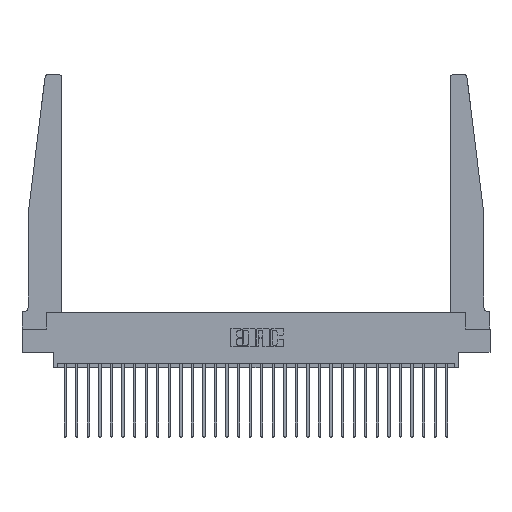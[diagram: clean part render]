
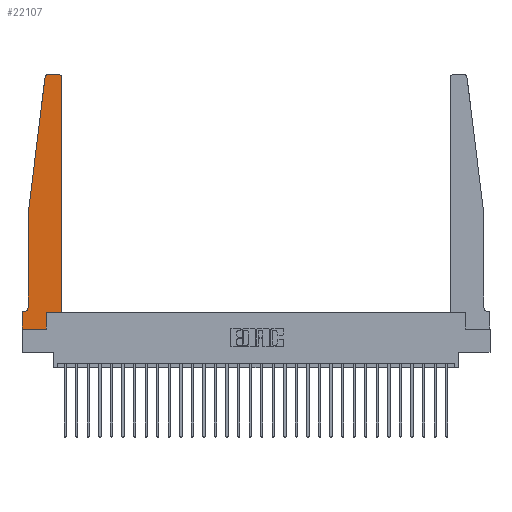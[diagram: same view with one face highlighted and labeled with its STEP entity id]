
A CAD part, top view. The second image highlights one B-rep face of the part: STEP entity #22107.
In plain terms, the highlighted planar face has unit normal (0, 0, 1).
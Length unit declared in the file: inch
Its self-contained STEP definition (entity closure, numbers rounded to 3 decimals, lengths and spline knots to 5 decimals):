
#262 = VERTEX_POINT ( 'NONE', #21662 ) ;
#724 = DIRECTION ( 'NONE',  ( 0., 0., -1. ) ) ;
#1283 = VECTOR ( 'NONE', #9118, 39.37008 ) ;
#1319 = CARTESIAN_POINT ( 'NONE',  ( 0.425, 0.18, 0.37 ) ) ;
#1551 = VECTOR ( 'NONE', #20176, 39.37008 ) ;
#1653 = CIRCLE ( 'NONE', #17897, 0.03 ) ;
#2287 = CARTESIAN_POINT ( 'NONE',  ( 0.425, 0.18, 0.37 ) ) ;
#2623 = EDGE_CURVE ( 'NONE', #11223, #9878, #7058, .T. ) ;
#3074 = ORIENTED_EDGE ( 'NONE', *, *, #16276, .T. ) ;
#3439 = LINE ( 'NONE', #27932, #18527 ) ;
#3899 = VERTEX_POINT ( 'NONE', #20298 ) ;
#3923 = CARTESIAN_POINT ( 'NONE',  ( 0.065, 1.25, 0.37 ) ) ;
#4147 = FACE_OUTER_BOUND ( 'NONE', #27017, .T. ) ;
#4292 = DIRECTION ( 'NONE',  ( -1., 0., 0. ) ) ;
#4382 = VECTOR ( 'NONE', #28266, 39.37008 ) ;
#4562 = VECTOR ( 'NONE', #27119, 39.37008 ) ;
#4894 = EDGE_CURVE ( 'NONE', #3899, #12848, #21574, .T. ) ;
#5672 = ORIENTED_EDGE ( 'NONE', *, *, #16887, .T. ) ;
#5782 = ORIENTED_EDGE ( 'NONE', *, *, #15178, .T. ) ;
#6183 = EDGE_CURVE ( 'NONE', #27841, #262, #23790, .T. ) ;
#6618 = CARTESIAN_POINT ( 'NONE',  ( 0., 0.1875, 0.37 ) ) ;
#7058 = CIRCLE ( 'NONE', #11235, 0.03 ) ;
#7682 = DIRECTION ( 'NONE',  ( -1., 0., 0. ) ) ;
#8371 = VERTEX_POINT ( 'NONE', #23908 ) ;
#8520 = PLANE ( 'NONE',  #11350 ) ;
#8958 = DIRECTION ( 'NONE',  ( 0., -1., 0. ) ) ;
#9078 = CARTESIAN_POINT ( 'NONE',  ( 0.27653, 2.75, 0.37 ) ) ;
#9118 = DIRECTION ( 'NONE',  ( 0., 1., 0. ) ) ;
#9304 = EDGE_CURVE ( 'NONE', #8371, #27841, #22900, .T. ) ;
#9561 = ORIENTED_EDGE ( 'NONE', *, *, #9304, .T. ) ;
#9772 = CARTESIAN_POINT ( 'NONE',  ( 0.015, 0.1875, 0.37 ) ) ;
#9878 = VERTEX_POINT ( 'NONE', #20741 ) ;
#10248 = ORIENTED_EDGE ( 'NONE', *, *, #12047, .T. ) ;
#10390 = ORIENTED_EDGE ( 'NONE', *, *, #2623, .T. ) ;
#10441 = CARTESIAN_POINT ( 'NONE',  ( 0.065, 0.1875, 0.37 ) ) ;
#10687 = ORIENTED_EDGE ( 'NONE', *, *, #6183, .T. ) ;
#10747 = VERTEX_POINT ( 'NONE', #9772 ) ;
#11015 = LINE ( 'NONE', #20310, #1283 ) ;
#11223 = VERTEX_POINT ( 'NONE', #21425 ) ;
#11235 = AXIS2_PLACEMENT_3D ( 'NONE', #19677, #15317, #24129 ) ;
#11350 = AXIS2_PLACEMENT_3D ( 'NONE', #6618, #28498, #13300 ) ;
#11377 = DIRECTION ( 'NONE',  ( 1., 0., 0. ) ) ;
#12047 = EDGE_CURVE ( 'NONE', #10747, #3899, #12605, .T. ) ;
#12605 = LINE ( 'NONE', #10441, #19700 ) ;
#12848 = VERTEX_POINT ( 'NONE', #27855 ) ;
#13276 = VECTOR ( 'NONE', #14287, 39.37008 ) ;
#13300 = DIRECTION ( 'NONE',  ( 1., 0., 0. ) ) ;
#13582 = CARTESIAN_POINT ( 'NONE',  ( 0.2605, 0.18, 0.37 ) ) ;
#14234 = VERTEX_POINT ( 'NONE', #28041 ) ;
#14240 = CARTESIAN_POINT ( 'NONE',  ( 0.015, 0.2375, 0.37 ) ) ;
#14287 = DIRECTION ( 'NONE',  ( 1., 0., 0. ) ) ;
#14784 = EDGE_CURVE ( 'NONE', #24383, #11223, #15962, .T. ) ;
#14974 = CARTESIAN_POINT ( 'NONE',  ( 0.425, 0.18, 0.37 ) ) ;
#15178 = EDGE_CURVE ( 'NONE', #9878, #27952, #19710, .T. ) ;
#15317 = DIRECTION ( 'NONE',  ( 0., 0., 1. ) ) ;
#15343 = CARTESIAN_POINT ( 'NONE',  ( 0.25, 2.75, 0.37 ) ) ;
#15627 = ORIENTED_EDGE ( 'NONE', *, *, #14784, .T. ) ;
#15761 = ORIENTED_EDGE ( 'NONE', *, *, #4894, .T. ) ;
#15962 = LINE ( 'NONE', #2287, #1551 ) ;
#15974 = ORIENTED_EDGE ( 'NONE', *, *, #23287, .T. ) ;
#16276 = EDGE_CURVE ( 'NONE', #27952, #8371, #1653, .T. ) ;
#16887 = EDGE_CURVE ( 'NONE', #262, #10747, #23474, .T. ) ;
#17201 = EDGE_CURVE ( 'NONE', #14234, #18966, #11015, .T. ) ;
#17897 = AXIS2_PLACEMENT_3D ( 'NONE', #26702, #22779, #11377 ) ;
#17973 = ORIENTED_EDGE ( 'NONE', *, *, #22774, .T. ) ;
#18527 = VECTOR ( 'NONE', #25624, 39.37008 ) ;
#18966 = VERTEX_POINT ( 'NONE', #13582 ) ;
#19677 = CARTESIAN_POINT ( 'NONE',  ( 0.395, 2.72, 0.37 ) ) ;
#19700 = VECTOR ( 'NONE', #21444, 39.37008 ) ;
#19710 = LINE ( 'NONE', #15343, #21905 ) ;
#20176 = DIRECTION ( 'NONE',  ( 0., 1., 0. ) ) ;
#20298 = CARTESIAN_POINT ( 'NONE',  ( 0., 0.1875, 0.37 ) ) ;
#20310 = CARTESIAN_POINT ( 'NONE',  ( 0.2605, 0.18, 0.37 ) ) ;
#20741 = CARTESIAN_POINT ( 'NONE',  ( 0.395, 2.75, 0.37 ) ) ;
#20755 = AXIS2_PLACEMENT_3D ( 'NONE', #14240, #724, #7682 ) ;
#21425 = CARTESIAN_POINT ( 'NONE',  ( 0.425, 2.72, 0.37 ) ) ;
#21444 = DIRECTION ( 'NONE',  ( -1., 0., 0. ) ) ;
#21574 = LINE ( 'NONE', #21713, #24575 ) ;
#21662 = CARTESIAN_POINT ( 'NONE',  ( 0.065, 0.2375, 0.37 ) ) ;
#21713 = CARTESIAN_POINT ( 'NONE',  ( 0., 0., 0.37 ) ) ;
#21882 = ORIENTED_EDGE ( 'NONE', *, *, #17201, .T. ) ;
#21905 = VECTOR ( 'NONE', #4292, 39.37008 ) ;
#22107 = ADVANCED_FACE ( 'NONE', ( #4147 ), #8520, .T. ) ;
#22774 = EDGE_CURVE ( 'NONE', #18966, #24383, #27586, .T. ) ;
#22779 = DIRECTION ( 'NONE',  ( 0., 0., 1. ) ) ;
#22900 = LINE ( 'NONE', #25102, #4562 ) ;
#23287 = EDGE_CURVE ( 'NONE', #12848, #14234, #3439, .T. ) ;
#23474 = CIRCLE ( 'NONE', #20755, 0.05 ) ;
#23790 = LINE ( 'NONE', #3923, #4382 ) ;
#23908 = CARTESIAN_POINT ( 'NONE',  ( 0.24675, 2.72367, 0.37 ) ) ;
#24129 = DIRECTION ( 'NONE',  ( 1., 0., 0. ) ) ;
#24383 = VERTEX_POINT ( 'NONE', #1319 ) ;
#24437 = CARTESIAN_POINT ( 'NONE',  ( 0.065, 1.25, 0.37 ) ) ;
#24575 = VECTOR ( 'NONE', #8958, 39.37008 ) ;
#25102 = CARTESIAN_POINT ( 'NONE',  ( 0.065, 1.25, 0.37 ) ) ;
#25624 = DIRECTION ( 'NONE',  ( 1., 0., 0. ) ) ;
#26702 = CARTESIAN_POINT ( 'NONE',  ( 0.27653, 2.72, 0.37 ) ) ;
#27017 = EDGE_LOOP ( 'NONE', ( #5782, #3074, #9561, #10687, #5672, #10248, #15761, #15974, #21882, #17973, #15627, #10390 ) ) ;
#27119 = DIRECTION ( 'NONE',  ( -0.122, -0.992, 0. ) ) ;
#27586 = LINE ( 'NONE', #14974, #13276 ) ;
#27841 = VERTEX_POINT ( 'NONE', #24437 ) ;
#27855 = CARTESIAN_POINT ( 'NONE',  ( 0., 0., 0.37 ) ) ;
#27932 = CARTESIAN_POINT ( 'NONE',  ( 0., 0., 0.37 ) ) ;
#27952 = VERTEX_POINT ( 'NONE', #9078 ) ;
#28041 = CARTESIAN_POINT ( 'NONE',  ( 0.2605, 0., 0.37 ) ) ;
#28266 = DIRECTION ( 'NONE',  ( 0., -1., 0. ) ) ;
#28498 = DIRECTION ( 'NONE',  ( 0., 0., 1. ) ) ;
